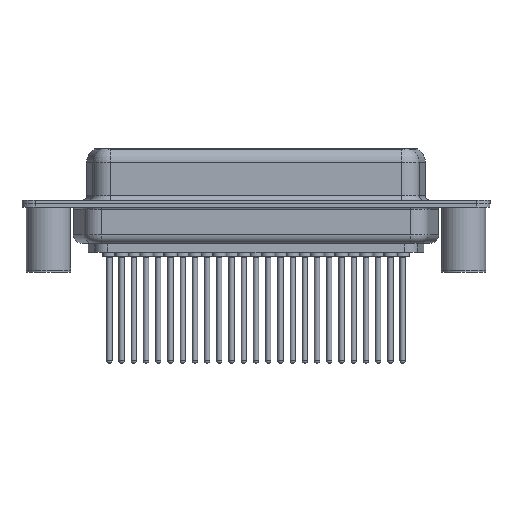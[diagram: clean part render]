
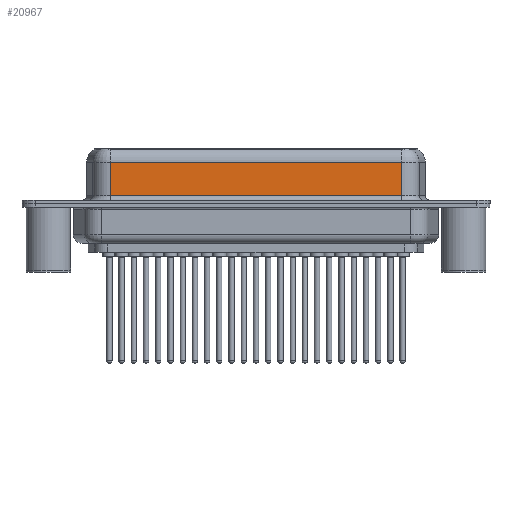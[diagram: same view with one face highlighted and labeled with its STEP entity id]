
A CAD part, front view. The second image highlights one B-rep face of the part: STEP entity #20967.
In plain terms, the highlighted planar face has unit normal (0, -1, 0).
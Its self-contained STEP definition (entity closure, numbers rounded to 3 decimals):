
#303 = EDGE_LOOP ( 'NONE', ( #16632, #7859, #21016, #19393 ) ) ;
#658 = DIRECTION ( 'NONE',  ( 0., 0., -1. ) ) ;
#1501 = VERTEX_POINT ( 'NONE', #17883 ) ;
#2169 = AXIS2_PLACEMENT_3D ( 'NONE', #6093, #14502, #7547 ) ;
#2238 = VECTOR ( 'NONE', #8759, 1000. ) ;
#2321 = FACE_OUTER_BOUND ( 'NONE', #303, .T. ) ;
#4378 = LINE ( 'NONE', #11090, #21231 ) ;
#4598 = CARTESIAN_POINT ( 'NONE',  ( 7.013, -3.95, 0.9 ) ) ;
#5181 = VECTOR ( 'NONE', #658, 1000. ) ;
#5456 = DIRECTION ( 'NONE',  ( 1., 0., 0. ) ) ;
#6093 = CARTESIAN_POINT ( 'NONE',  ( 40.037, -3.95, 6.4 ) ) ;
#6138 = LINE ( 'NONE', #19790, #5181 ) ;
#6393 = LINE ( 'NONE', #13313, #2238 ) ;
#6669 = CARTESIAN_POINT ( 'NONE',  ( 7.013, -3.95, 4.65 ) ) ;
#7547 = DIRECTION ( 'NONE',  ( 0., 0., 1. ) ) ;
#7859 = ORIENTED_EDGE ( 'NONE', *, *, #22154, .T. ) ;
#8759 = DIRECTION ( 'NONE',  ( -1., 0., 0. ) ) ;
#9497 = DIRECTION ( 'NONE',  ( 0., 0., -1. ) ) ;
#10003 = VECTOR ( 'NONE', #5456, 1000. ) ;
#10778 = CARTESIAN_POINT ( 'NONE',  ( 40.037, -3.95, 0.9 ) ) ;
#11090 = CARTESIAN_POINT ( 'NONE',  ( 7.013, -3.95, 6.4 ) ) ;
#11318 = PLANE ( 'NONE',  #2169 ) ;
#12774 = EDGE_CURVE ( 'NONE', #1501, #17074, #6138, .T. ) ;
#13313 = CARTESIAN_POINT ( 'NONE',  ( 40.037, -3.95, 4.65 ) ) ;
#14502 = DIRECTION ( 'NONE',  ( 0., 1., 0. ) ) ;
#14966 = EDGE_CURVE ( 'NONE', #19069, #21130, #4378, .T. ) ;
#15580 = EDGE_CURVE ( 'NONE', #21130, #17074, #21018, .T. ) ;
#16037 = CARTESIAN_POINT ( 'NONE',  ( 40.037, -3.95, 0.9 ) ) ;
#16632 = ORIENTED_EDGE ( 'NONE', *, *, #12774, .F. ) ;
#17074 = VERTEX_POINT ( 'NONE', #16037 ) ;
#17883 = CARTESIAN_POINT ( 'NONE',  ( 40.037, -3.95, 4.65 ) ) ;
#19069 = VERTEX_POINT ( 'NONE', #6669 ) ;
#19393 = ORIENTED_EDGE ( 'NONE', *, *, #15580, .T. ) ;
#19790 = CARTESIAN_POINT ( 'NONE',  ( 40.037, -3.95, 6.4 ) ) ;
#20967 = ADVANCED_FACE ( 'NONE', ( #2321 ), #11318, .F. ) ;
#21016 = ORIENTED_EDGE ( 'NONE', *, *, #14966, .T. ) ;
#21018 = LINE ( 'NONE', #10778, #10003 ) ;
#21130 = VERTEX_POINT ( 'NONE', #4598 ) ;
#21231 = VECTOR ( 'NONE', #9497, 1000. ) ;
#22154 = EDGE_CURVE ( 'NONE', #1501, #19069, #6393, .T. ) ;
